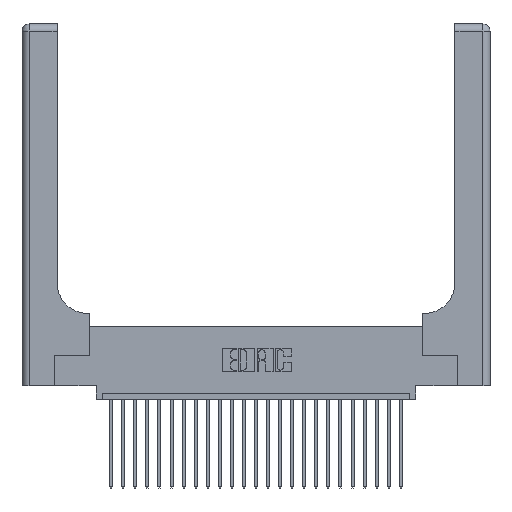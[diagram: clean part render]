
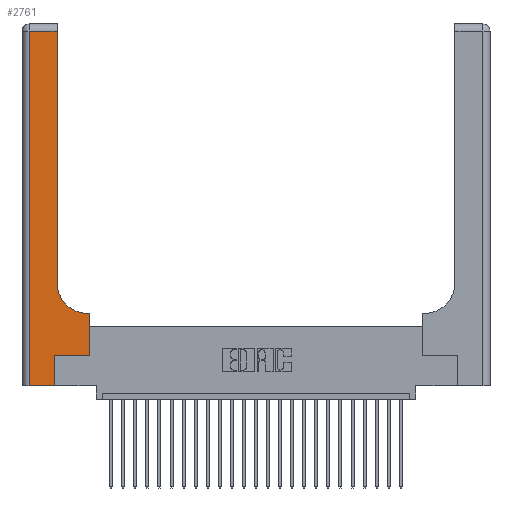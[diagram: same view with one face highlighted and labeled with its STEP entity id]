
A CAD part, top view. The second image highlights one B-rep face of the part: STEP entity #2761.
In plain terms, the highlighted planar face has unit normal (0, 0, 1).
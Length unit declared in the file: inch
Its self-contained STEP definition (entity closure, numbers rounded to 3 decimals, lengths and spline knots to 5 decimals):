
#322 = VERTEX_POINT ( 'NONE', #9981 ) ;
#857 = PLANE ( 'NONE',  #9593 ) ;
#965 = VERTEX_POINT ( 'NONE', #7620 ) ;
#1173 = VERTEX_POINT ( 'NONE', #3633 ) ;
#1350 = EDGE_LOOP ( 'NONE', ( #19633, #16312, #5972, #2460, #7595, #11041, #3515, #9980, #2854 ) ) ;
#1582 = DIRECTION ( 'NONE',  ( 1., 0., 0. ) ) ;
#1755 = LINE ( 'NONE', #26125, #3095 ) ;
#1783 = VECTOR ( 'NONE', #12742, 39.37008 ) ;
#1965 = VECTOR ( 'NONE', #5026, 39.37008 ) ;
#2048 = CARTESIAN_POINT ( 'NONE',  ( 0.06, 2.94, 0.37 ) ) ;
#2429 = LINE ( 'NONE', #10610, #1783 ) ;
#2460 = ORIENTED_EDGE ( 'NONE', *, *, #25016, .T. ) ;
#2761 = ADVANCED_FACE ( 'NONE', ( #7903 ), #857, .F. ) ;
#2854 = ORIENTED_EDGE ( 'NONE', *, *, #8846, .T. ) ;
#3095 = VECTOR ( 'NONE', #1582, 39.37008 ) ;
#3515 = ORIENTED_EDGE ( 'NONE', *, *, #20835, .T. ) ;
#3633 = CARTESIAN_POINT ( 'NONE',  ( 0.2915, 0.85, 0.37 ) ) ;
#4822 = CARTESIAN_POINT ( 'NONE',  ( 0., 3., 0.37 ) ) ;
#4888 = VECTOR ( 'NONE', #12574, 39.37008 ) ;
#4892 = DIRECTION ( 'NONE',  ( 1., 0., 0. ) ) ;
#5026 = DIRECTION ( 'NONE',  ( 0., 1., 0. ) ) ;
#5713 = CARTESIAN_POINT ( 'NONE',  ( 0., 2.94, 0.37 ) ) ;
#5925 = LINE ( 'NONE', #5713, #14567 ) ;
#5972 = ORIENTED_EDGE ( 'NONE', *, *, #13008, .T. ) ;
#6416 = CARTESIAN_POINT ( 'NONE',  ( 0., 0., 0.37 ) ) ;
#6473 = LINE ( 'NONE', #6416, #4888 ) ;
#7595 = ORIENTED_EDGE ( 'NONE', *, *, #22766, .T. ) ;
#7620 = CARTESIAN_POINT ( 'NONE',  ( 0.5585, 0.6, 0.37 ) ) ;
#7903 = FACE_OUTER_BOUND ( 'NONE', #1350, .T. ) ;
#8820 = DIRECTION ( 'NONE',  ( 0., 1., 0. ) ) ;
#8846 = EDGE_CURVE ( 'NONE', #13061, #1173, #20352, .T. ) ;
#8919 = DIRECTION ( 'NONE',  ( -1., 0., 0. ) ) ;
#8993 = AXIS2_PLACEMENT_3D ( 'NONE', #21488, #17221, #4892 ) ;
#9453 = DIRECTION ( 'NONE',  ( 0., -1., 0. ) ) ;
#9593 = AXIS2_PLACEMENT_3D ( 'NONE', #4822, #13125, #8919 ) ;
#9980 = ORIENTED_EDGE ( 'NONE', *, *, #18541, .T. ) ;
#9981 = CARTESIAN_POINT ( 'NONE',  ( 0.06, 0., 0.37 ) ) ;
#10610 = CARTESIAN_POINT ( 'NONE',  ( 0.2915, 0.6, 0.37 ) ) ;
#10865 = VERTEX_POINT ( 'NONE', #2048 ) ;
#11041 = ORIENTED_EDGE ( 'NONE', *, *, #22531, .T. ) ;
#11822 = VECTOR ( 'NONE', #9453, 39.37008 ) ;
#11982 = DIRECTION ( 'NONE',  ( -1., 0., 0. ) ) ;
#12574 = DIRECTION ( 'NONE',  ( 1., 0., 0. ) ) ;
#12742 = DIRECTION ( 'NONE',  ( -1., 0., 0. ) ) ;
#12988 = LINE ( 'NONE', #18926, #15559 ) ;
#13008 = EDGE_CURVE ( 'NONE', #10865, #322, #17244, .T. ) ;
#13061 = VERTEX_POINT ( 'NONE', #22198 ) ;
#13125 = DIRECTION ( 'NONE',  ( 0., 0., -1. ) ) ;
#14097 = VERTEX_POINT ( 'NONE', #16271 ) ;
#14567 = VECTOR ( 'NONE', #11982, 39.37008 ) ;
#15181 = EDGE_CURVE ( 'NONE', #1173, #19919, #23865, .T. ) ;
#15467 = CARTESIAN_POINT ( 'NONE',  ( 0.5585, 0.25, 0.37 ) ) ;
#15559 = VECTOR ( 'NONE', #8820, 39.37008 ) ;
#16195 = VECTOR ( 'NONE', #23898, 39.37008 ) ;
#16271 = CARTESIAN_POINT ( 'NONE',  ( 0.269, 0., 0.37 ) ) ;
#16312 = ORIENTED_EDGE ( 'NONE', *, *, #22602, .T. ) ;
#17221 = DIRECTION ( 'NONE',  ( 0., 0., -1. ) ) ;
#17244 = LINE ( 'NONE', #21495, #11822 ) ;
#17724 = CARTESIAN_POINT ( 'NONE',  ( 0.2915, 3., 0.37 ) ) ;
#18541 = EDGE_CURVE ( 'NONE', #965, #13061, #2429, .T. ) ;
#18926 = CARTESIAN_POINT ( 'NONE',  ( 0.269, 0., 0.37 ) ) ;
#19633 = ORIENTED_EDGE ( 'NONE', *, *, #15181, .T. ) ;
#19919 = VERTEX_POINT ( 'NONE', #20093 ) ;
#20093 = CARTESIAN_POINT ( 'NONE',  ( 0.2915, 2.94, 0.37 ) ) ;
#20352 = CIRCLE ( 'NONE', #8993, 0.25 ) ;
#20835 = EDGE_CURVE ( 'NONE', #24688, #965, #26235, .T. ) ;
#21488 = CARTESIAN_POINT ( 'NONE',  ( 0.5415, 0.85, 0.37 ) ) ;
#21495 = CARTESIAN_POINT ( 'NONE',  ( 0.06, 3., 0.37 ) ) ;
#22198 = CARTESIAN_POINT ( 'NONE',  ( 0.5415, 0.6, 0.37 ) ) ;
#22531 = EDGE_CURVE ( 'NONE', #24092, #24688, #1755, .T. ) ;
#22602 = EDGE_CURVE ( 'NONE', #19919, #10865, #5925, .T. ) ;
#22766 = EDGE_CURVE ( 'NONE', #14097, #24092, #12988, .T. ) ;
#22966 = CARTESIAN_POINT ( 'NONE',  ( 0.269, 0.25, 0.37 ) ) ;
#23865 = LINE ( 'NONE', #17724, #16195 ) ;
#23898 = DIRECTION ( 'NONE',  ( 0., 1., 0. ) ) ;
#24092 = VERTEX_POINT ( 'NONE', #22966 ) ;
#24688 = VERTEX_POINT ( 'NONE', #15467 ) ;
#25016 = EDGE_CURVE ( 'NONE', #322, #14097, #6473, .T. ) ;
#25261 = CARTESIAN_POINT ( 'NONE',  ( 0.5585, 0.25, 0.37 ) ) ;
#26125 = CARTESIAN_POINT ( 'NONE',  ( 0.269, 0.25, 0.37 ) ) ;
#26235 = LINE ( 'NONE', #25261, #1965 ) ;
